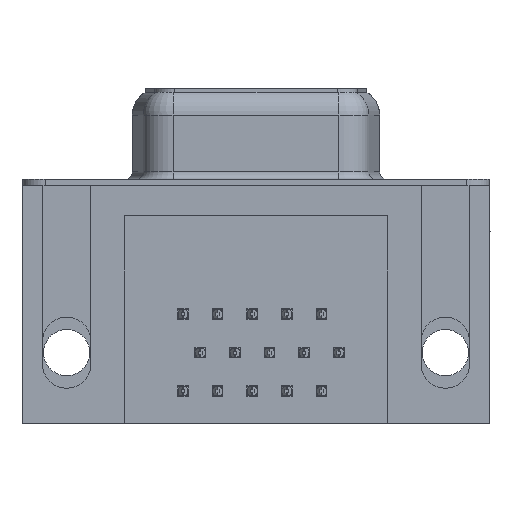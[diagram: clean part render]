
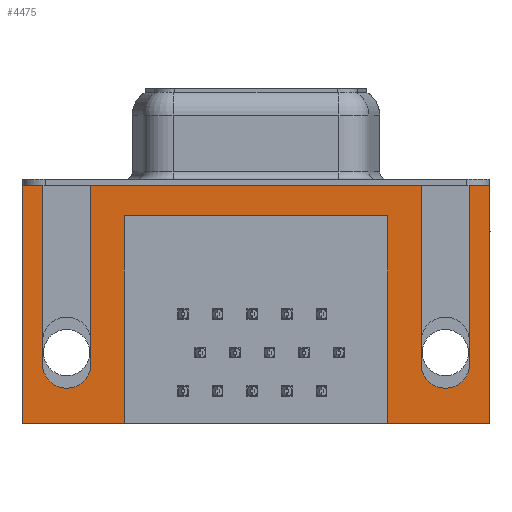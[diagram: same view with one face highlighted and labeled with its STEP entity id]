
A CAD part, front view. The second image highlights one B-rep face of the part: STEP entity #4475.
In plain terms, the highlighted planar face has unit normal (0, -1, 0).
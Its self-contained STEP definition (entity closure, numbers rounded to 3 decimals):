
#202 = CARTESIAN_POINT ( 'NONE',  ( 21.2, -6.275, -2. ) ) ;
#251 = CARTESIAN_POINT ( 'NONE',  ( -1.6, -6.275, -11.78 ) ) ;
#823 = ORIENTED_EDGE ( 'NONE', *, *, #5856, .F. ) ;
#1707 = LINE ( 'NONE', #15901, #31263 ) ;
#1956 = EDGE_CURVE ( 'NONE', #12302, #12680, #3465, .T. ) ;
#2953 = ORIENTED_EDGE ( 'NONE', *, *, #4480, .F. ) ;
#3167 = EDGE_CURVE ( 'NONE', #31561, #22115, #33837, .T. ) ;
#3358 = VECTOR ( 'NONE', #22772, 1000. ) ;
#3408 = EDGE_CURVE ( 'NONE', #33019, #6027, #32366, .T. ) ;
#3465 = LINE ( 'NONE', #32797, #3358 ) ;
#4181 = CARTESIAN_POINT ( 'NONE',  ( 26.59, -6.275, 0. ) ) ;
#4475 = ADVANCED_FACE ( 'NONE', ( #24546 ), #32951, .T. ) ;
#4479 = DIRECTION ( 'NONE',  ( 0., 0., 1. ) ) ;
#4480 = EDGE_CURVE ( 'NONE', #11119, #31561, #24670, .T. ) ;
#4534 = VERTEX_POINT ( 'NONE', #18889 ) ;
#4946 = VERTEX_POINT ( 'NONE', #21075 ) ;
#5609 = LINE ( 'NONE', #29897, #20759 ) ;
#5759 = LINE ( 'NONE', #31691, #5944 ) ;
#5856 = EDGE_CURVE ( 'NONE', #6027, #11119, #16886, .T. ) ;
#5904 = ORIENTED_EDGE ( 'NONE', *, *, #7832, .F. ) ;
#5944 = VECTOR ( 'NONE', #11689, 1000. ) ;
#6027 = VERTEX_POINT ( 'NONE', #17647 ) ;
#6797 = CIRCLE ( 'NONE', #34208, 1.6 ) ;
#7359 = ORIENTED_EDGE ( 'NONE', *, *, #26957, .F. ) ;
#7832 = EDGE_CURVE ( 'NONE', #11944, #33019, #5759, .T. ) ;
#8538 = AXIS2_PLACEMENT_3D ( 'NONE', #27216, #10184, #30127 ) ;
#9072 = CARTESIAN_POINT ( 'NONE',  ( 27.9, -6.275, -2.5 ) ) ;
#9578 = EDGE_CURVE ( 'NONE', #12680, #35520, #28739, .T. ) ;
#9838 = CARTESIAN_POINT ( 'NONE',  ( -1.6, -6.275, 0. ) ) ;
#10184 = DIRECTION ( 'NONE',  ( 0., -1., 0. ) ) ;
#10448 = CARTESIAN_POINT ( 'NONE',  ( 3.79, -6.275, -2. ) ) ;
#11068 = CARTESIAN_POINT ( 'NONE',  ( 23.39, -6.275, 0. ) ) ;
#11119 = VERTEX_POINT ( 'NONE', #33556 ) ;
#11200 = ORIENTED_EDGE ( 'NONE', *, *, #1956, .F. ) ;
#11341 = AXIS2_PLACEMENT_3D ( 'NONE', #15663, #35844, #18519 ) ;
#11689 = DIRECTION ( 'NONE',  ( 0., 0., 1. ) ) ;
#11892 = LINE ( 'NONE', #202, #19382 ) ;
#11944 = VERTEX_POINT ( 'NONE', #21526 ) ;
#11993 = CARTESIAN_POINT ( 'NONE',  ( -1.6, -6.275, 0. ) ) ;
#12302 = VERTEX_POINT ( 'NONE', #20987 ) ;
#12471 = CARTESIAN_POINT ( 'NONE',  ( 27.9, -6.275, -15.7 ) ) ;
#12680 = VERTEX_POINT ( 'NONE', #11993 ) ;
#12773 = DIRECTION ( 'NONE',  ( 1., 0., 0. ) ) ;
#12777 = EDGE_CURVE ( 'NONE', #33192, #25359, #19261, .T. ) ;
#13007 = VECTOR ( 'NONE', #21504, 1000. ) ;
#13032 = DIRECTION ( 'NONE',  ( 0., -1., 0. ) ) ;
#13130 = ORIENTED_EDGE ( 'NONE', *, *, #12777, .F. ) ;
#13235 = DIRECTION ( 'NONE',  ( 0., 0., -1. ) ) ;
#14437 = EDGE_CURVE ( 'NONE', #4946, #33192, #24637, .T. ) ;
#14563 = CARTESIAN_POINT ( 'NONE',  ( 26.59, -6.275, 0. ) ) ;
#15259 = DIRECTION ( 'NONE',  ( -1., 0., 0. ) ) ;
#15385 = ORIENTED_EDGE ( 'NONE', *, *, #14437, .F. ) ;
#15663 = CARTESIAN_POINT ( 'NONE',  ( -2.91, -6.275, -2.5 ) ) ;
#15802 = CARTESIAN_POINT ( 'NONE',  ( 27.9, -6.275, 0. ) ) ;
#15879 = EDGE_CURVE ( 'NONE', #19632, #4946, #1707, .T. ) ;
#15901 = CARTESIAN_POINT ( 'NONE',  ( 3.79, -6.275, -2. ) ) ;
#15916 = DIRECTION ( 'NONE',  ( 0., 0., -1. ) ) ;
#16886 = LINE ( 'NONE', #11068, #16992 ) ;
#16992 = VECTOR ( 'NONE', #28096, 1000. ) ;
#17647 = CARTESIAN_POINT ( 'NONE',  ( 23.39, -6.275, 0. ) ) ;
#18189 = LINE ( 'NONE', #9072, #24140 ) ;
#18191 = DIRECTION ( 'NONE',  ( -1., 0., 0. ) ) ;
#18285 = ORIENTED_EDGE ( 'NONE', *, *, #9578, .F. ) ;
#18316 = CARTESIAN_POINT ( 'NONE',  ( 1.6, -6.275, 0. ) ) ;
#18519 = DIRECTION ( 'NONE',  ( 0., 0., -1. ) ) ;
#18551 = CARTESIAN_POINT ( 'NONE',  ( -2.91, -6.275, -2.5 ) ) ;
#18889 = CARTESIAN_POINT ( 'NONE',  ( 27.9, -6.275, -15.7 ) ) ;
#18981 = VECTOR ( 'NONE', #18191, 1000. ) ;
#19261 = LINE ( 'NONE', #12471, #26032 ) ;
#19382 = VECTOR ( 'NONE', #31170, 1000. ) ;
#19622 = VERTEX_POINT ( 'NONE', #15802 ) ;
#19632 = VERTEX_POINT ( 'NONE', #35978 ) ;
#20424 = EDGE_CURVE ( 'NONE', #32380, #19632, #11892, .T. ) ;
#20759 = VECTOR ( 'NONE', #12773, 1000. ) ;
#20987 = CARTESIAN_POINT ( 'NONE',  ( -2.91, -6.275, 0. ) ) ;
#21075 = CARTESIAN_POINT ( 'NONE',  ( 3.79, -6.275, -2. ) ) ;
#21338 = ORIENTED_EDGE ( 'NONE', *, *, #20424, .F. ) ;
#21504 = DIRECTION ( 'NONE',  ( 0., 0., 1. ) ) ;
#21511 = LINE ( 'NONE', #18551, #13007 ) ;
#21526 = CARTESIAN_POINT ( 'NONE',  ( 1.6, -6.275, -11.78 ) ) ;
#21685 = EDGE_CURVE ( 'NONE', #4534, #32380, #34358, .T. ) ;
#22115 = VERTEX_POINT ( 'NONE', #14563 ) ;
#22151 = CARTESIAN_POINT ( 'NONE',  ( 26.59, -6.275, -11.78 ) ) ;
#22772 = DIRECTION ( 'NONE',  ( 1., 0., 0. ) ) ;
#22889 = CARTESIAN_POINT ( 'NONE',  ( 3.79, -6.275, -15.7 ) ) ;
#23176 = ORIENTED_EDGE ( 'NONE', *, *, #33775, .T. ) ;
#24140 = VECTOR ( 'NONE', #26080, 1000. ) ;
#24546 = FACE_OUTER_BOUND ( 'NONE', #26115, .T. ) ;
#24637 = LINE ( 'NONE', #10448, #33222 ) ;
#24670 = CIRCLE ( 'NONE', #8538, 1.6 ) ;
#25359 = VERTEX_POINT ( 'NONE', #27003 ) ;
#25465 = CARTESIAN_POINT ( 'NONE',  ( -2.91, -6.275, 0. ) ) ;
#26032 = VECTOR ( 'NONE', #15259, 1000. ) ;
#26080 = DIRECTION ( 'NONE',  ( 0., 0., 1. ) ) ;
#26115 = EDGE_LOOP ( 'NONE', ( #34296, #2953, #823, #26972, #5904, #34144, #18285, #11200, #7359, #13130, #15385, #31980, #21338, #32990, #23176, #31636 ) ) ;
#26957 = EDGE_CURVE ( 'NONE', #25359, #12302, #21511, .T. ) ;
#26972 = ORIENTED_EDGE ( 'NONE', *, *, #3408, .F. ) ;
#27003 = CARTESIAN_POINT ( 'NONE',  ( -2.91, -6.275, -15.7 ) ) ;
#27216 = CARTESIAN_POINT ( 'NONE',  ( 24.99, -6.275, -11.78 ) ) ;
#28096 = DIRECTION ( 'NONE',  ( 0., 0., -1. ) ) ;
#28739 = LINE ( 'NONE', #9838, #28768 ) ;
#28768 = VECTOR ( 'NONE', #15916, 1000. ) ;
#29897 = CARTESIAN_POINT ( 'NONE',  ( -2.91, -6.275, 0. ) ) ;
#30108 = CARTESIAN_POINT ( 'NONE',  ( 21.2, -6.275, -15.7 ) ) ;
#30127 = DIRECTION ( 'NONE',  ( -1., 0., 0. ) ) ;
#30185 = CARTESIAN_POINT ( 'NONE',  ( 0., -6.275, -11.78 ) ) ;
#30925 = DIRECTION ( 'NONE',  ( 1., 0., 0. ) ) ;
#31170 = DIRECTION ( 'NONE',  ( 0., 0., 1. ) ) ;
#31263 = VECTOR ( 'NONE', #36085, 1000. ) ;
#31561 = VERTEX_POINT ( 'NONE', #22151 ) ;
#31636 = ORIENTED_EDGE ( 'NONE', *, *, #37223, .F. ) ;
#31691 = CARTESIAN_POINT ( 'NONE',  ( 1.6, -6.275, 0. ) ) ;
#31980 = ORIENTED_EDGE ( 'NONE', *, *, #15879, .F. ) ;
#32366 = LINE ( 'NONE', #25465, #32805 ) ;
#32380 = VERTEX_POINT ( 'NONE', #30108 ) ;
#32513 = CARTESIAN_POINT ( 'NONE',  ( 27.9, -6.275, -15.7 ) ) ;
#32797 = CARTESIAN_POINT ( 'NONE',  ( -2.91, -6.275, 0. ) ) ;
#32805 = VECTOR ( 'NONE', #30925, 1000. ) ;
#32951 = PLANE ( 'NONE',  #11341 ) ;
#32990 = ORIENTED_EDGE ( 'NONE', *, *, #21685, .F. ) ;
#33019 = VERTEX_POINT ( 'NONE', #18316 ) ;
#33029 = EDGE_CURVE ( 'NONE', #35520, #11944, #6797, .T. ) ;
#33138 = DIRECTION ( 'NONE',  ( 1., 0., 0. ) ) ;
#33192 = VERTEX_POINT ( 'NONE', #22889 ) ;
#33222 = VECTOR ( 'NONE', #13235, 1000. ) ;
#33556 = CARTESIAN_POINT ( 'NONE',  ( 23.39, -6.275, -11.78 ) ) ;
#33726 = VECTOR ( 'NONE', #4479, 1000. ) ;
#33775 = EDGE_CURVE ( 'NONE', #4534, #19622, #18189, .T. ) ;
#33837 = LINE ( 'NONE', #4181, #33726 ) ;
#34144 = ORIENTED_EDGE ( 'NONE', *, *, #33029, .F. ) ;
#34208 = AXIS2_PLACEMENT_3D ( 'NONE', #30185, #13032, #33138 ) ;
#34296 = ORIENTED_EDGE ( 'NONE', *, *, #3167, .F. ) ;
#34358 = LINE ( 'NONE', #32513, #18981 ) ;
#35520 = VERTEX_POINT ( 'NONE', #251 ) ;
#35844 = DIRECTION ( 'NONE',  ( 0., -1., 0. ) ) ;
#35978 = CARTESIAN_POINT ( 'NONE',  ( 21.2, -6.275, -2. ) ) ;
#36085 = DIRECTION ( 'NONE',  ( -1., 0., 0. ) ) ;
#37223 = EDGE_CURVE ( 'NONE', #22115, #19622, #5609, .T. ) ;
